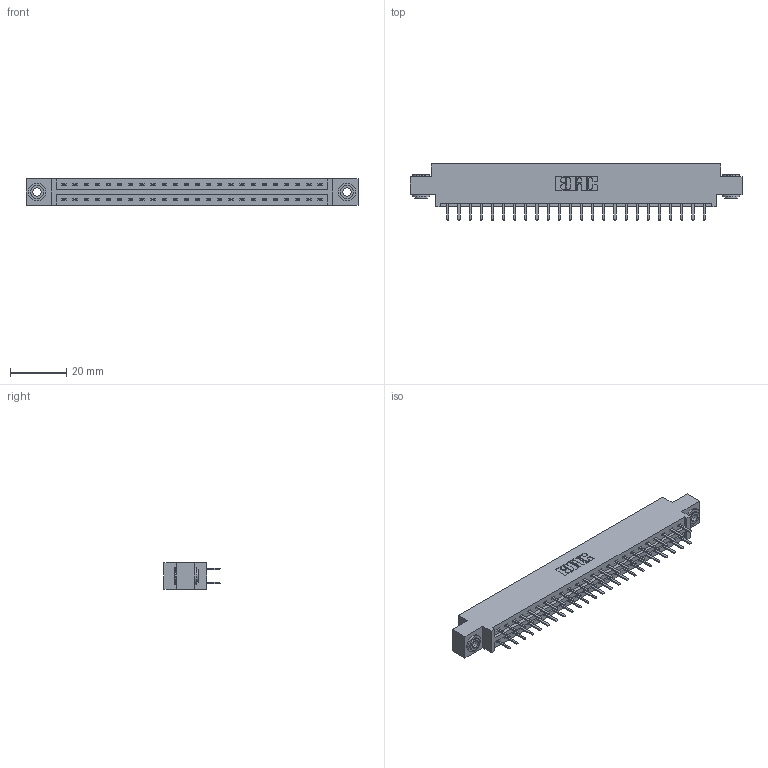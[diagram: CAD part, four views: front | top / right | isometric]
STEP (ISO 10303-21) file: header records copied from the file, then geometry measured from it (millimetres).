
FILE_DESCRIPTION (( 'STEP AP203' ), '1' );
FILE_NAME ('387-048-520-803.STEP', '2019-10-18T09:00:24', ( '' ), ( '' ), 'SwSTEP 2.0', 'SolidWorks 2016', '' );
FILE_SCHEMA (( 'CONFIG_CONTROL_DESIGN' ));
Length unit declared in the file: inch
Products named in the file (4): 387-048-520-803; 345-250-002_345-250-002-102; 345-292-001_345-293-120; 337 Part_0.170 Offset - 0.156 Dia-TH
Assembly tree (51 placements, depth 2):
  387-048-520-803
    337 Part_0.170 Offset - 0.156 Dia-TH
    345-292-001_345-293-120  x48
    345-250-002_345-250-002-102  x2
Bounding box: 118.11 x 20.02 x 9.4 mm (x, y, z)
Volume: 12088.6 mm3; surface area: 13763.3 mm2
Topology: 51 solids, 51 shells, 2940 faces, 8511 edges, 5542 vertices
Faces by surface type: plane 2004, cylinder 928, cone 8
Entity records: 21832 total; most frequent: CARTESIAN_POINT 3681, ORIENTED_EDGE 3598, DIRECTION 3185, EDGE_CURVE 1799, LINE 1643, VECTOR 1643, VERTEX_POINT 1194, AXIS2_PLACEMENT_3D 771
